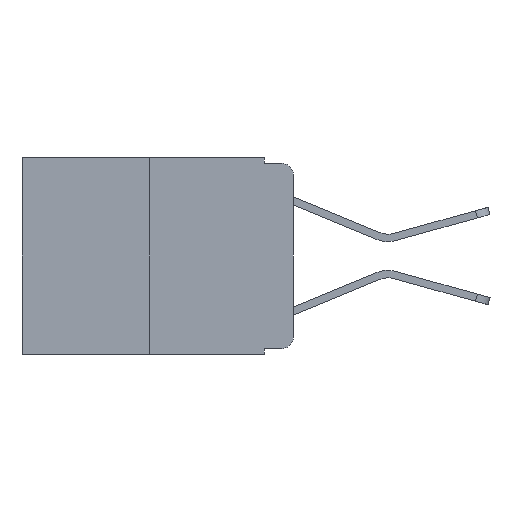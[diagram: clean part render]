
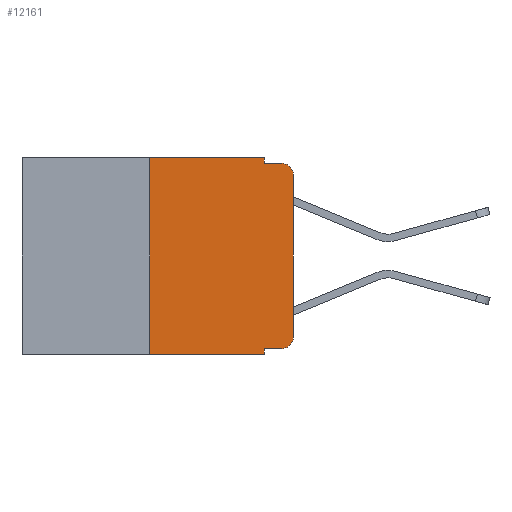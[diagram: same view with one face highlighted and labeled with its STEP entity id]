
A CAD part, left-side view. The second image highlights one B-rep face of the part: STEP entity #12161.
In plain terms, the highlighted planar face has unit normal (-1, 0, 0).
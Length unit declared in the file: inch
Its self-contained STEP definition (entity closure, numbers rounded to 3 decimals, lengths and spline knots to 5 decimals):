
#18 = LINE ( 'NONE', #1774, #11946 ) ;
#112 = ORIENTED_EDGE ( 'NONE', *, *, #1051, .F. ) ;
#353 = ORIENTED_EDGE ( 'NONE', *, *, #13509, .F. ) ;
#398 = CARTESIAN_POINT ( 'NONE',  ( 0., 0.02, -0.03 ) ) ;
#515 = ORIENTED_EDGE ( 'NONE', *, *, #3842, .T. ) ;
#1051 = EDGE_CURVE ( 'NONE', #3230, #13115, #18, .T. ) ;
#1167 = ORIENTED_EDGE ( 'NONE', *, *, #8327, .T. ) ;
#1304 = FACE_OUTER_BOUND ( 'NONE', #12715, .T. ) ;
#1427 = DIRECTION ( 'NONE',  ( 0., 0., -1. ) ) ;
#1574 = DIRECTION ( 'NONE',  ( 0., 0., -1. ) ) ;
#1774 = CARTESIAN_POINT ( 'NONE',  ( 0., 0.051, 0. ) ) ;
#1867 = DIRECTION ( 'NONE',  ( 0., 0., -1. ) ) ;
#1920 = ORIENTED_EDGE ( 'NONE', *, *, #7643, .T. ) ;
#2089 = VERTEX_POINT ( 'NONE', #11314 ) ;
#2296 = LINE ( 'NONE', #9370, #13100 ) ;
#3203 = CARTESIAN_POINT ( 'NONE',  ( 0., 0.25, 0. ) ) ;
#3230 = VERTEX_POINT ( 'NONE', #9656 ) ;
#3236 = VERTEX_POINT ( 'NONE', #10134 ) ;
#3842 = EDGE_CURVE ( 'NONE', #7088, #9158, #12515, .T. ) ;
#3884 = CIRCLE ( 'NONE', #10821, 0.02 ) ;
#3961 = CARTESIAN_POINT ( 'NONE',  ( 0., 0.473, 0. ) ) ;
#4095 = CARTESIAN_POINT ( 'NONE',  ( 0., 0., -0.03 ) ) ;
#4316 = EDGE_CURVE ( 'NONE', #8000, #3236, #11190, .T. ) ;
#4367 = ORIENTED_EDGE ( 'NONE', *, *, #13205, .T. ) ;
#4456 = PLANE ( 'NONE',  #4733 ) ;
#4612 = LINE ( 'NONE', #3961, #11132 ) ;
#4733 = AXIS2_PLACEMENT_3D ( 'NONE', #13052, #6869, #4837 ) ;
#4786 = CARTESIAN_POINT ( 'NONE',  ( 0., 0.02, -0.313 ) ) ;
#4837 = DIRECTION ( 'NONE',  ( 0., 0., -1. ) ) ;
#5155 = DIRECTION ( 'NONE',  ( 0., -1., 0. ) ) ;
#5356 = CARTESIAN_POINT ( 'NONE',  ( 0., 0.051, -0.01 ) ) ;
#5411 = DIRECTION ( 'NONE',  ( 0., -1., 0. ) ) ;
#5855 = VECTOR ( 'NONE', #5155, 39.37008 ) ;
#5856 = VECTOR ( 'NONE', #5411, 39.37008 ) ;
#6143 = CARTESIAN_POINT ( 'NONE',  ( 0., 0., -0.313 ) ) ;
#6322 = VECTOR ( 'NONE', #12487, 39.37008 ) ;
#6480 = ORIENTED_EDGE ( 'NONE', *, *, #10293, .F. ) ;
#6869 = DIRECTION ( 'NONE',  ( 1., 0., 0. ) ) ;
#7088 = VERTEX_POINT ( 'NONE', #4095 ) ;
#7534 = LINE ( 'NONE', #11564, #5855 ) ;
#7567 = CARTESIAN_POINT ( 'NONE',  ( 0., 0., 0. ) ) ;
#7643 = EDGE_CURVE ( 'NONE', #10287, #3236, #9848, .T. ) ;
#7765 = DIRECTION ( 'NONE',  ( -1., 0., 0. ) ) ;
#7791 = ORIENTED_EDGE ( 'NONE', *, *, #9494, .F. ) ;
#8000 = VERTEX_POINT ( 'NONE', #9243 ) ;
#8269 = DIRECTION ( 'NONE',  ( 0., -1., 0. ) ) ;
#8327 = EDGE_CURVE ( 'NONE', #8857, #7088, #11357, .T. ) ;
#8623 = DIRECTION ( 'NONE',  ( 0., 0., 1. ) ) ;
#8857 = VERTEX_POINT ( 'NONE', #6143 ) ;
#8917 = DIRECTION ( 'NONE',  ( -1., 0., 0. ) ) ;
#9156 = VECTOR ( 'NONE', #8623, 39.37008 ) ;
#9158 = VERTEX_POINT ( 'NONE', #10201 ) ;
#9243 = CARTESIAN_POINT ( 'NONE',  ( 0., 0.051, -0.333 ) ) ;
#9370 = CARTESIAN_POINT ( 'NONE',  ( 0., 0.051, -0.333 ) ) ;
#9494 = EDGE_CURVE ( 'NONE', #10287, #2089, #12145, .T. ) ;
#9633 = CARTESIAN_POINT ( 'NONE',  ( 0., 0.473, -0.343 ) ) ;
#9656 = CARTESIAN_POINT ( 'NONE',  ( 0., 0.051, 0. ) ) ;
#9703 = VERTEX_POINT ( 'NONE', #11544 ) ;
#9848 = LINE ( 'NONE', #9633, #5856 ) ;
#10067 = ORIENTED_EDGE ( 'NONE', *, *, #11111, .T. ) ;
#10134 = CARTESIAN_POINT ( 'NONE',  ( 0., 0.051, -0.343 ) ) ;
#10201 = CARTESIAN_POINT ( 'NONE',  ( 0., 0.02, -0.01 ) ) ;
#10287 = VERTEX_POINT ( 'NONE', #13275 ) ;
#10293 = EDGE_CURVE ( 'NONE', #2089, #3230, #4612, .T. ) ;
#10371 = DIRECTION ( 'NONE',  ( 0., -1., 0. ) ) ;
#10637 = AXIS2_PLACEMENT_3D ( 'NONE', #398, #7765, #1427 ) ;
#10821 = AXIS2_PLACEMENT_3D ( 'NONE', #4786, #8917, #1574 ) ;
#11066 = ORIENTED_EDGE ( 'NONE', *, *, #4316, .F. ) ;
#11111 = EDGE_CURVE ( 'NONE', #8000, #9703, #2296, .T. ) ;
#11132 = VECTOR ( 'NONE', #10371, 39.37008 ) ;
#11190 = LINE ( 'NONE', #11523, #6322 ) ;
#11314 = CARTESIAN_POINT ( 'NONE',  ( 0., 0.25, 0. ) ) ;
#11357 = LINE ( 'NONE', #7567, #9156 ) ;
#11523 = CARTESIAN_POINT ( 'NONE',  ( 0., 0.051, 0. ) ) ;
#11544 = CARTESIAN_POINT ( 'NONE',  ( 0., 0.02, -0.333 ) ) ;
#11564 = CARTESIAN_POINT ( 'NONE',  ( 0., 0.051, -0.01 ) ) ;
#11946 = VECTOR ( 'NONE', #1867, 39.37008 ) ;
#12145 = LINE ( 'NONE', #3203, #12478 ) ;
#12161 = ADVANCED_FACE ( 'NONE', ( #1304 ), #4456, .F. ) ;
#12478 = VECTOR ( 'NONE', #12673, 39.37008 ) ;
#12487 = DIRECTION ( 'NONE',  ( 0., 0., -1. ) ) ;
#12515 = CIRCLE ( 'NONE', #10637, 0.02 ) ;
#12673 = DIRECTION ( 'NONE',  ( 0., 0., 1. ) ) ;
#12715 = EDGE_LOOP ( 'NONE', ( #1167, #515, #353, #112, #6480, #7791, #1920, #11066, #10067, #4367 ) ) ;
#13052 = CARTESIAN_POINT ( 'NONE',  ( 0., 0.473, 0. ) ) ;
#13100 = VECTOR ( 'NONE', #8269, 39.37008 ) ;
#13115 = VERTEX_POINT ( 'NONE', #5356 ) ;
#13205 = EDGE_CURVE ( 'NONE', #9703, #8857, #3884, .T. ) ;
#13275 = CARTESIAN_POINT ( 'NONE',  ( 0., 0.25, -0.343 ) ) ;
#13509 = EDGE_CURVE ( 'NONE', #13115, #9158, #7534, .T. ) ;
